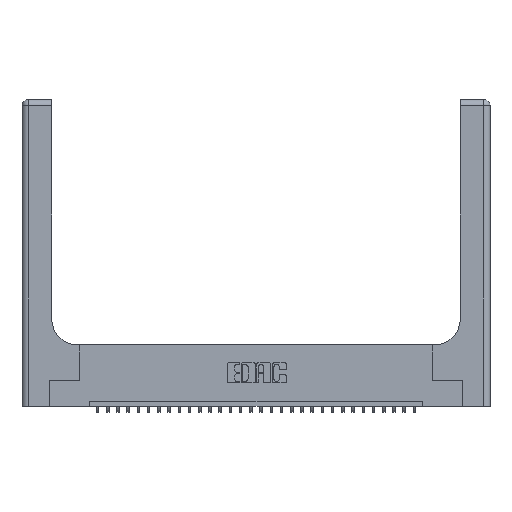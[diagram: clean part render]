
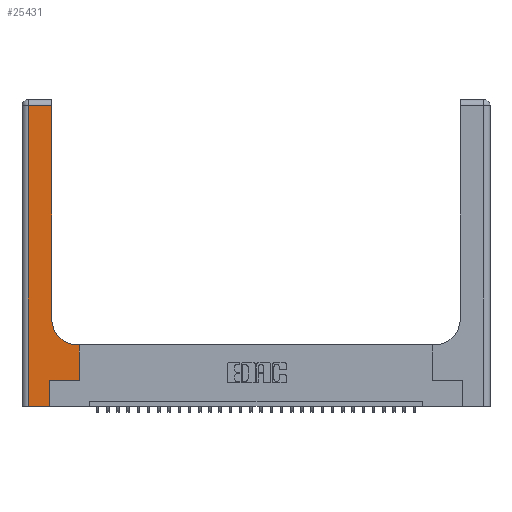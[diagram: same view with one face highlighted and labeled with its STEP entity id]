
A CAD part, top view. The second image highlights one B-rep face of the part: STEP entity #25431.
In plain terms, the highlighted planar face has unit normal (0, 0, 1).
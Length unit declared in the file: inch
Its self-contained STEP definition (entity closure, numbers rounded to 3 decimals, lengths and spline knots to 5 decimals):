
#114 = EDGE_CURVE ( 'NONE', #12548, #5698, #30119, .T. ) ;
#130 = DIRECTION ( 'NONE',  ( 1., 0., 0. ) ) ;
#272 = CARTESIAN_POINT ( 'NONE',  ( 0.2915, 3., 0.37 ) ) ;
#323 = VERTEX_POINT ( 'NONE', #11550 ) ;
#421 = CARTESIAN_POINT ( 'NONE',  ( 0.269, 0., 0.37 ) ) ;
#444 = PLANE ( 'NONE',  #15505 ) ;
#882 = LINE ( 'NONE', #2763, #6851 ) ;
#1151 = EDGE_CURVE ( 'NONE', #17209, #29474, #11858, .T. ) ;
#2003 = DIRECTION ( 'NONE',  ( -1., 0., 0. ) ) ;
#2018 = CARTESIAN_POINT ( 'NONE',  ( 0.06, 2.94, 0.37 ) ) ;
#2673 = CARTESIAN_POINT ( 'NONE',  ( 0.5585, 0.6, 0.37 ) ) ;
#2763 = CARTESIAN_POINT ( 'NONE',  ( 0.5585, 0.25, 0.37 ) ) ;
#3514 = CARTESIAN_POINT ( 'NONE',  ( 0.5585, 0.25, 0.37 ) ) ;
#4661 = CARTESIAN_POINT ( 'NONE',  ( 0.06, 3., 0.37 ) ) ;
#4728 = CARTESIAN_POINT ( 'NONE',  ( 0., 2.94, 0.37 ) ) ;
#5698 = VERTEX_POINT ( 'NONE', #20748 ) ;
#5911 = LINE ( 'NONE', #26159, #13275 ) ;
#5938 = LINE ( 'NONE', #4661, #12955 ) ;
#6044 = ORIENTED_EDGE ( 'NONE', *, *, #7400, .T. ) ;
#6140 = ORIENTED_EDGE ( 'NONE', *, *, #1151, .T. ) ;
#6460 = CARTESIAN_POINT ( 'NONE',  ( 0.5415, 0.85, 0.37 ) ) ;
#6851 = VECTOR ( 'NONE', #16636, 39.37008 ) ;
#7272 = EDGE_CURVE ( 'NONE', #13054, #18757, #29302, .T. ) ;
#7336 = ORIENTED_EDGE ( 'NONE', *, *, #25637, .T. ) ;
#7400 = EDGE_CURVE ( 'NONE', #14162, #13054, #20379, .T. ) ;
#7896 = LINE ( 'NONE', #272, #27915 ) ;
#8624 = DIRECTION ( 'NONE',  ( 1., 0., 0. ) ) ;
#8892 = VECTOR ( 'NONE', #2003, 39.37008 ) ;
#10770 = VERTEX_POINT ( 'NONE', #2673 ) ;
#11243 = ORIENTED_EDGE ( 'NONE', *, *, #25683, .T. ) ;
#11464 = CARTESIAN_POINT ( 'NONE',  ( 0.269, 0.25, 0.37 ) ) ;
#11550 = CARTESIAN_POINT ( 'NONE',  ( 0.06, 0., 0.37 ) ) ;
#11858 = LINE ( 'NONE', #4728, #8892 ) ;
#12548 = VERTEX_POINT ( 'NONE', #22330 ) ;
#12955 = VECTOR ( 'NONE', #13627, 39.37008 ) ;
#13054 = VERTEX_POINT ( 'NONE', #19759 ) ;
#13077 = LINE ( 'NONE', #16462, #25698 ) ;
#13275 = VECTOR ( 'NONE', #130, 39.37008 ) ;
#13627 = DIRECTION ( 'NONE',  ( 0., -1., 0. ) ) ;
#13697 = CARTESIAN_POINT ( 'NONE',  ( 0.2915, 2.94, 0.37 ) ) ;
#14162 = VERTEX_POINT ( 'NONE', #421 ) ;
#14413 = VECTOR ( 'NONE', #26773, 39.37008 ) ;
#15316 = FACE_OUTER_BOUND ( 'NONE', #20222, .T. ) ;
#15505 = AXIS2_PLACEMENT_3D ( 'NONE', #28533, #23786, #24007 ) ;
#15762 = DIRECTION ( 'NONE',  ( 0., 0., -1. ) ) ;
#16462 = CARTESIAN_POINT ( 'NONE',  ( 0.2915, 0.6, 0.37 ) ) ;
#16636 = DIRECTION ( 'NONE',  ( 0., 1., 0. ) ) ;
#17209 = VERTEX_POINT ( 'NONE', #13697 ) ;
#18641 = DIRECTION ( 'NONE',  ( 1., 0., 0. ) ) ;
#18757 = VERTEX_POINT ( 'NONE', #3514 ) ;
#19153 = EDGE_CURVE ( 'NONE', #18757, #10770, #882, .T. ) ;
#19759 = CARTESIAN_POINT ( 'NONE',  ( 0.269, 0.25, 0.37 ) ) ;
#20222 = EDGE_LOOP ( 'NONE', ( #7336, #6140, #28586, #23660, #6044, #28366, #24966, #11243, #25197 ) ) ;
#20379 = LINE ( 'NONE', #21566, #14413 ) ;
#20748 = CARTESIAN_POINT ( 'NONE',  ( 0.2915, 0.85, 0.37 ) ) ;
#21523 = EDGE_CURVE ( 'NONE', #29474, #323, #5938, .T. ) ;
#21566 = CARTESIAN_POINT ( 'NONE',  ( 0.269, 0., 0.37 ) ) ;
#22198 = EDGE_CURVE ( 'NONE', #323, #14162, #5911, .T. ) ;
#22330 = CARTESIAN_POINT ( 'NONE',  ( 0.5415, 0.6, 0.37 ) ) ;
#22886 = AXIS2_PLACEMENT_3D ( 'NONE', #6460, #15762, #8624 ) ;
#23660 = ORIENTED_EDGE ( 'NONE', *, *, #22198, .T. ) ;
#23786 = DIRECTION ( 'NONE',  ( 0., 0., -1. ) ) ;
#24007 = DIRECTION ( 'NONE',  ( -1., 0., 0. ) ) ;
#24966 = ORIENTED_EDGE ( 'NONE', *, *, #19153, .T. ) ;
#25197 = ORIENTED_EDGE ( 'NONE', *, *, #114, .T. ) ;
#25431 = ADVANCED_FACE ( 'NONE', ( #15316 ), #444, .F. ) ;
#25637 = EDGE_CURVE ( 'NONE', #5698, #17209, #7896, .T. ) ;
#25683 = EDGE_CURVE ( 'NONE', #10770, #12548, #13077, .T. ) ;
#25698 = VECTOR ( 'NONE', #30724, 39.37008 ) ;
#26159 = CARTESIAN_POINT ( 'NONE',  ( 0., 0., 0.37 ) ) ;
#26773 = DIRECTION ( 'NONE',  ( 0., 1., 0. ) ) ;
#27779 = VECTOR ( 'NONE', #18641, 39.37008 ) ;
#27915 = VECTOR ( 'NONE', #28661, 39.37008 ) ;
#28366 = ORIENTED_EDGE ( 'NONE', *, *, #7272, .T. ) ;
#28533 = CARTESIAN_POINT ( 'NONE',  ( 0., 3., 0.37 ) ) ;
#28586 = ORIENTED_EDGE ( 'NONE', *, *, #21523, .T. ) ;
#28661 = DIRECTION ( 'NONE',  ( 0., 1., 0. ) ) ;
#29302 = LINE ( 'NONE', #11464, #27779 ) ;
#29474 = VERTEX_POINT ( 'NONE', #2018 ) ;
#30119 = CIRCLE ( 'NONE', #22886, 0.25 ) ;
#30724 = DIRECTION ( 'NONE',  ( -1., 0., 0. ) ) ;
